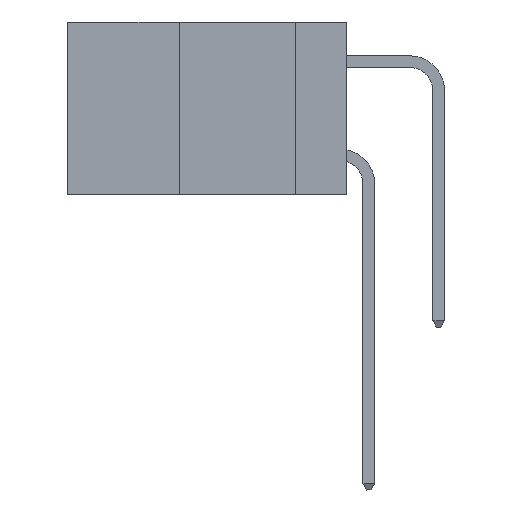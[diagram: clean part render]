
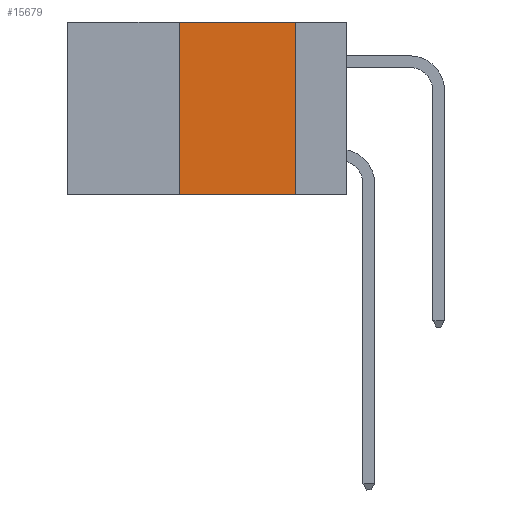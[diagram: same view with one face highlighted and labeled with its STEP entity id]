
A CAD part, left-side view. The second image highlights one B-rep face of the part: STEP entity #15679.
In plain terms, the highlighted planar face has unit normal (-1, 0, 0).
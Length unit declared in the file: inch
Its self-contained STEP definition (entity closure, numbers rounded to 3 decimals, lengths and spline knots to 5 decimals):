
#39 = VECTOR ( 'NONE', #16732, 39.37008 ) ;
#518 = ORIENTED_EDGE ( 'NONE', *, *, #15882, .F. ) ;
#934 = VERTEX_POINT ( 'NONE', #19371 ) ;
#1218 = ORIENTED_EDGE ( 'NONE', *, *, #19744, .F. ) ;
#1245 = CARTESIAN_POINT ( 'NONE',  ( 0., 0.6, 0. ) ) ;
#1260 = CARTESIAN_POINT ( 'NONE',  ( 0., 0.11, 0. ) ) ;
#1645 = ORIENTED_EDGE ( 'NONE', *, *, #15643, .T. ) ;
#3032 = DIRECTION ( 'NONE',  ( 0., 0., -1. ) ) ;
#3514 = CARTESIAN_POINT ( 'NONE',  ( 0., 0.11, -0.37 ) ) ;
#4350 = AXIS2_PLACEMENT_3D ( 'NONE', #1245, #12423, #3032 ) ;
#7440 = CARTESIAN_POINT ( 'NONE',  ( 0., 0.11, 0. ) ) ;
#8294 = VERTEX_POINT ( 'NONE', #1260 ) ;
#8862 = VECTOR ( 'NONE', #19706, 39.37008 ) ;
#8902 = LINE ( 'NONE', #19782, #39 ) ;
#9401 = PLANE ( 'NONE',  #4350 ) ;
#10923 = VECTOR ( 'NONE', #12353, 39.37008 ) ;
#11134 = LINE ( 'NONE', #12880, #14725 ) ;
#12353 = DIRECTION ( 'NONE',  ( 0., -1., 0. ) ) ;
#12423 = DIRECTION ( 'NONE',  ( 1., 0., 0. ) ) ;
#12559 = EDGE_CURVE ( 'NONE', #8294, #18864, #12867, .T. ) ;
#12867 = LINE ( 'NONE', #7440, #8862 ) ;
#12880 = CARTESIAN_POINT ( 'NONE',  ( 0., 0.6, 0. ) ) ;
#14407 = DIRECTION ( 'NONE',  ( 0., -1., 0. ) ) ;
#14480 = FACE_OUTER_BOUND ( 'NONE', #15548, .T. ) ;
#14554 = VERTEX_POINT ( 'NONE', #15629 ) ;
#14725 = VECTOR ( 'NONE', #14407, 39.37008 ) ;
#14990 = LINE ( 'NONE', #15386, #10923 ) ;
#15386 = CARTESIAN_POINT ( 'NONE',  ( 0., 0.6, -0.37 ) ) ;
#15548 = EDGE_LOOP ( 'NONE', ( #16930, #518, #1218, #1645 ) ) ;
#15629 = CARTESIAN_POINT ( 'NONE',  ( 0., 0.36, 0. ) ) ;
#15643 = EDGE_CURVE ( 'NONE', #934, #18864, #14990, .T. ) ;
#15679 = ADVANCED_FACE ( 'NONE', ( #14480 ), #9401, .F. ) ;
#15882 = EDGE_CURVE ( 'NONE', #14554, #8294, #11134, .T. ) ;
#16732 = DIRECTION ( 'NONE',  ( 0., 0., 1. ) ) ;
#16930 = ORIENTED_EDGE ( 'NONE', *, *, #12559, .F. ) ;
#18864 = VERTEX_POINT ( 'NONE', #3514 ) ;
#19371 = CARTESIAN_POINT ( 'NONE',  ( 0., 0.36, -0.37 ) ) ;
#19706 = DIRECTION ( 'NONE',  ( 0., 0., -1. ) ) ;
#19744 = EDGE_CURVE ( 'NONE', #934, #14554, #8902, .T. ) ;
#19782 = CARTESIAN_POINT ( 'NONE',  ( 0., 0.36, 0. ) ) ;
